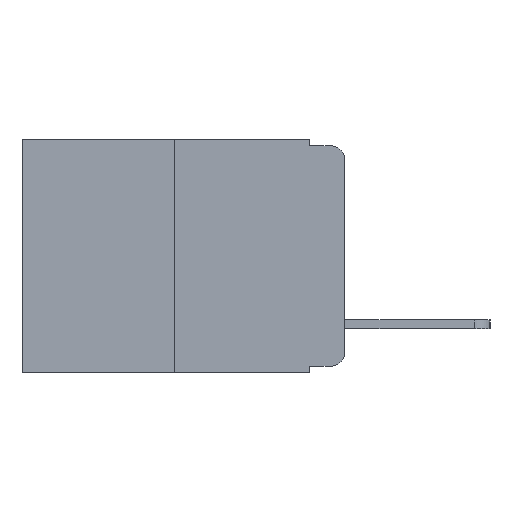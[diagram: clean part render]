
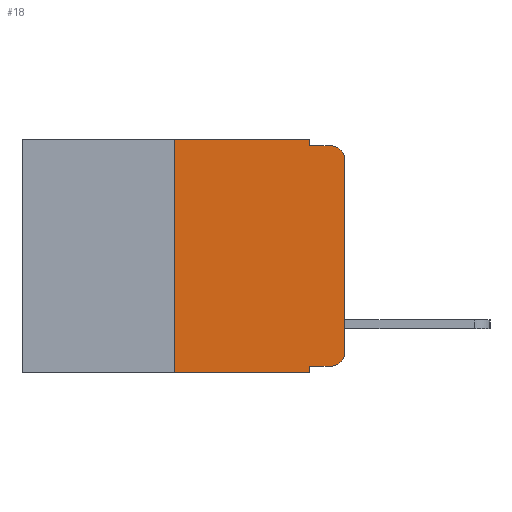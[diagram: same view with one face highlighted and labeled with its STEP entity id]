
A CAD part, left-side view. The second image highlights one B-rep face of the part: STEP entity #18.
In plain terms, the highlighted planar face has unit normal (-1, 0, 0).
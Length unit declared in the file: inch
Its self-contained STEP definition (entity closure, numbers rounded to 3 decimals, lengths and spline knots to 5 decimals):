
#18 = ADVANCED_FACE ( 'NONE', ( #6518 ), #962, .F. ) ;
#22 = CARTESIAN_POINT ( 'NONE',  ( 0., 0., 0. ) ) ;
#132 = CARTESIAN_POINT ( 'NONE',  ( 0., 0.473, 0. ) ) ;
#444 = LINE ( 'NONE', #8102, #12719 ) ;
#962 = PLANE ( 'NONE',  #1942 ) ;
#965 = LINE ( 'NONE', #11845, #9391 ) ;
#1741 = AXIS2_PLACEMENT_3D ( 'NONE', #5124, #15162, #6632 ) ;
#1942 = AXIS2_PLACEMENT_3D ( 'NONE', #132, #10499, #8283 ) ;
#2426 = CARTESIAN_POINT ( 'NONE',  ( 0., 0.051, -0.333 ) ) ;
#2824 = EDGE_CURVE ( 'NONE', #10451, #10710, #10959, .T. ) ;
#3788 = LINE ( 'NONE', #7226, #18243 ) ;
#3972 = CARTESIAN_POINT ( 'NONE',  ( 0., 0., -0.03 ) ) ;
#4514 = DIRECTION ( 'NONE',  ( 0., 0., -1. ) ) ;
#4525 = CARTESIAN_POINT ( 'NONE',  ( 0., 0.02, -0.01 ) ) ;
#5124 = CARTESIAN_POINT ( 'NONE',  ( 0., 0.02, -0.313 ) ) ;
#5192 = VECTOR ( 'NONE', #14980, 39.37008 ) ;
#5773 = EDGE_CURVE ( 'NONE', #15695, #11695, #444, .T. ) ;
#6017 = CARTESIAN_POINT ( 'NONE',  ( 0., 0.051, 0. ) ) ;
#6518 = FACE_OUTER_BOUND ( 'NONE', #7063, .T. ) ;
#6596 = DIRECTION ( 'NONE',  ( 0., 0., 1. ) ) ;
#6632 = DIRECTION ( 'NONE',  ( 0., 0., -1. ) ) ;
#7063 = EDGE_LOOP ( 'NONE', ( #7207, #7437, #7601, #7636, #7669, #7878, #8904, #8927, #9002, #9509 ) ) ;
#7207 = ORIENTED_EDGE ( 'NONE', *, *, #7715, .T. ) ;
#7226 = CARTESIAN_POINT ( 'NONE',  ( 0., 0.473, -0.343 ) ) ;
#7255 = VERTEX_POINT ( 'NONE', #11041 ) ;
#7437 = ORIENTED_EDGE ( 'NONE', *, *, #7682, .T. ) ;
#7543 = EDGE_CURVE ( 'NONE', #10856, #17518, #965, .T. ) ;
#7601 = ORIENTED_EDGE ( 'NONE', *, *, #12178, .F. ) ;
#7636 = ORIENTED_EDGE ( 'NONE', *, *, #2824, .F. ) ;
#7669 = ORIENTED_EDGE ( 'NONE', *, *, #16788, .F. ) ;
#7682 = EDGE_CURVE ( 'NONE', #18161, #13730, #13318, .T. ) ;
#7715 = EDGE_CURVE ( 'NONE', #15259, #18161, #11991, .T. ) ;
#7852 = DIRECTION ( 'NONE',  ( 0., -1., 0. ) ) ;
#7878 = ORIENTED_EDGE ( 'NONE', *, *, #7543, .F. ) ;
#7892 = VECTOR ( 'NONE', #10189, 39.37008 ) ;
#8052 = CARTESIAN_POINT ( 'NONE',  ( 0., 0.051, -0.01 ) ) ;
#8077 = CARTESIAN_POINT ( 'NONE',  ( 0., 0.02, -0.03 ) ) ;
#8102 = CARTESIAN_POINT ( 'NONE',  ( 0., 0.051, 0. ) ) ;
#8283 = DIRECTION ( 'NONE',  ( 0., 0., -1. ) ) ;
#8904 = ORIENTED_EDGE ( 'NONE', *, *, #18712, .T. ) ;
#8927 = ORIENTED_EDGE ( 'NONE', *, *, #5773, .F. ) ;
#9002 = ORIENTED_EDGE ( 'NONE', *, *, #9034, .T. ) ;
#9034 = EDGE_CURVE ( 'NONE', #15695, #7255, #18977, .T. ) ;
#9391 = VECTOR ( 'NONE', #14648, 39.37008 ) ;
#9509 = ORIENTED_EDGE ( 'NONE', *, *, #14697, .T. ) ;
#9518 = DIRECTION ( 'NONE',  ( 0., 0., -1. ) ) ;
#9688 = CIRCLE ( 'NONE', #1741, 0.02 ) ;
#9939 = CARTESIAN_POINT ( 'NONE',  ( 0., 0.25, -0.343 ) ) ;
#10189 = DIRECTION ( 'NONE',  ( 0., -1., 0. ) ) ;
#10451 = VERTEX_POINT ( 'NONE', #13070 ) ;
#10499 = DIRECTION ( 'NONE',  ( 1., 0., 0. ) ) ;
#10710 = VERTEX_POINT ( 'NONE', #16409 ) ;
#10856 = VERTEX_POINT ( 'NONE', #9939 ) ;
#10959 = LINE ( 'NONE', #6017, #18045 ) ;
#11041 = CARTESIAN_POINT ( 'NONE',  ( 0., 0.02, -0.333 ) ) ;
#11695 = VERTEX_POINT ( 'NONE', #14117 ) ;
#11845 = CARTESIAN_POINT ( 'NONE',  ( 0., 0.25, 0. ) ) ;
#11991 = LINE ( 'NONE', #22, #15711 ) ;
#12178 = EDGE_CURVE ( 'NONE', #10710, #13730, #13330, .T. ) ;
#12719 = VECTOR ( 'NONE', #16561, 39.37008 ) ;
#12977 = CARTESIAN_POINT ( 'NONE',  ( 0., 0.25, 0. ) ) ;
#13070 = CARTESIAN_POINT ( 'NONE',  ( 0., 0.051, 0. ) ) ;
#13318 = CIRCLE ( 'NONE', #15356, 0.02 ) ;
#13330 = LINE ( 'NONE', #8052, #5192 ) ;
#13469 = CARTESIAN_POINT ( 'NONE',  ( 0., 0.051, -0.333 ) ) ;
#13730 = VERTEX_POINT ( 'NONE', #4525 ) ;
#14117 = CARTESIAN_POINT ( 'NONE',  ( 0., 0.051, -0.343 ) ) ;
#14648 = DIRECTION ( 'NONE',  ( 0., 0., 1. ) ) ;
#14697 = EDGE_CURVE ( 'NONE', #7255, #15259, #9688, .T. ) ;
#14762 = VECTOR ( 'NONE', #7852, 39.37008 ) ;
#14980 = DIRECTION ( 'NONE',  ( 0., -1., 0. ) ) ;
#15162 = DIRECTION ( 'NONE',  ( -1., 0., 0. ) ) ;
#15259 = VERTEX_POINT ( 'NONE', #19362 ) ;
#15356 = AXIS2_PLACEMENT_3D ( 'NONE', #8077, #17965, #9518 ) ;
#15695 = VERTEX_POINT ( 'NONE', #2426 ) ;
#15711 = VECTOR ( 'NONE', #6596, 39.37008 ) ;
#16409 = CARTESIAN_POINT ( 'NONE',  ( 0., 0.051, -0.01 ) ) ;
#16561 = DIRECTION ( 'NONE',  ( 0., 0., -1. ) ) ;
#16788 = EDGE_CURVE ( 'NONE', #17518, #10451, #19138, .T. ) ;
#17219 = CARTESIAN_POINT ( 'NONE',  ( 0., 0.473, 0. ) ) ;
#17518 = VERTEX_POINT ( 'NONE', #12977 ) ;
#17965 = DIRECTION ( 'NONE',  ( -1., 0., 0. ) ) ;
#18045 = VECTOR ( 'NONE', #4514, 39.37008 ) ;
#18161 = VERTEX_POINT ( 'NONE', #3972 ) ;
#18243 = VECTOR ( 'NONE', #18586, 39.37008 ) ;
#18586 = DIRECTION ( 'NONE',  ( 0., -1., 0. ) ) ;
#18712 = EDGE_CURVE ( 'NONE', #10856, #11695, #3788, .T. ) ;
#18977 = LINE ( 'NONE', #13469, #14762 ) ;
#19138 = LINE ( 'NONE', #17219, #7892 ) ;
#19362 = CARTESIAN_POINT ( 'NONE',  ( 0., 0., -0.313 ) ) ;
